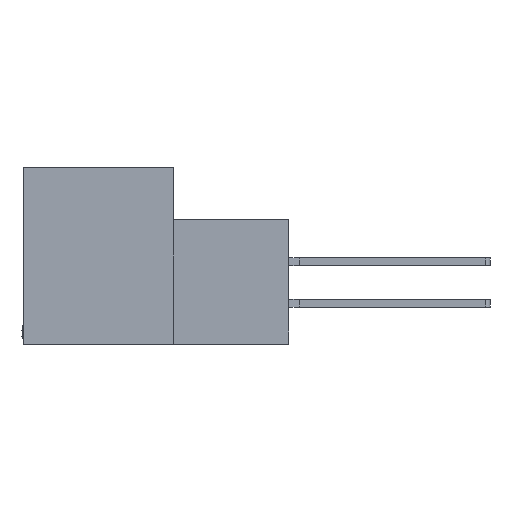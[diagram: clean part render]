
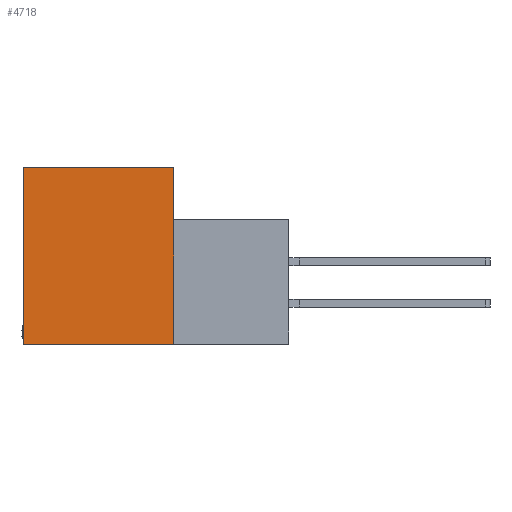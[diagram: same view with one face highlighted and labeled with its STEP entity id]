
A CAD part, left-side view. The second image highlights one B-rep face of the part: STEP entity #4718.
In plain terms, the highlighted planar face has unit normal (-1, 0, 0).
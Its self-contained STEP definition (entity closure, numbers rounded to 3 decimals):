
#235 = DIRECTION ( 'NONE',  ( 0., 0., 1. ) ) ;
#270 = VECTOR ( 'NONE', #8214, 1000. ) ;
#2529 = VERTEX_POINT ( 'NONE', #7531 ) ;
#2599 = AXIS2_PLACEMENT_3D ( 'NONE', #23667, #19995, #5098 ) ;
#4718 = ADVANCED_FACE ( 'NONE', ( #18733 ), #21499, .F. ) ;
#5098 = DIRECTION ( 'NONE',  ( 0., 0., -1. ) ) ;
#5476 = EDGE_CURVE ( 'NONE', #12645, #7682, #20450, .T. ) ;
#7056 = DIRECTION ( 'NONE',  ( 0., 1., 0. ) ) ;
#7314 = CARTESIAN_POINT ( 'NONE',  ( 0., 11.506, 0. ) ) ;
#7531 = CARTESIAN_POINT ( 'NONE',  ( 0., 11.506, -13.487 ) ) ;
#7675 = CARTESIAN_POINT ( 'NONE',  ( 0., 0., 0. ) ) ;
#7682 = VERTEX_POINT ( 'NONE', #7675 ) ;
#7828 = LINE ( 'NONE', #21684, #22513 ) ;
#8214 = DIRECTION ( 'NONE',  ( 0., -1., 0. ) ) ;
#8284 = CARTESIAN_POINT ( 'NONE',  ( 0., 11.506, 0. ) ) ;
#9219 = EDGE_LOOP ( 'NONE', ( #10697, #18334, #13505, #21819 ) ) ;
#9712 = CARTESIAN_POINT ( 'NONE',  ( 0., 0., 0. ) ) ;
#10315 = EDGE_CURVE ( 'NONE', #12982, #2529, #7828, .T. ) ;
#10697 = ORIENTED_EDGE ( 'NONE', *, *, #10315, .F. ) ;
#11489 = EDGE_CURVE ( 'NONE', #7682, #12982, #21360, .T. ) ;
#11737 = DIRECTION ( 'NONE',  ( 0., 0., -1. ) ) ;
#11888 = CARTESIAN_POINT ( 'NONE',  ( 0., 0., -13.487 ) ) ;
#12155 = VECTOR ( 'NONE', #11737, 1000. ) ;
#12645 = VERTEX_POINT ( 'NONE', #7314 ) ;
#12982 = VERTEX_POINT ( 'NONE', #11888 ) ;
#13505 = ORIENTED_EDGE ( 'NONE', *, *, #5476, .F. ) ;
#17398 = VECTOR ( 'NONE', #235, 1000. ) ;
#17971 = LINE ( 'NONE', #20854, #17398 ) ;
#18334 = ORIENTED_EDGE ( 'NONE', *, *, #11489, .F. ) ;
#18733 = FACE_OUTER_BOUND ( 'NONE', #9219, .T. ) ;
#19995 = DIRECTION ( 'NONE',  ( 1., 0., 0. ) ) ;
#20450 = LINE ( 'NONE', #8284, #270 ) ;
#20854 = CARTESIAN_POINT ( 'NONE',  ( 0., 11.506, -13.487 ) ) ;
#21169 = EDGE_CURVE ( 'NONE', #2529, #12645, #17971, .T. ) ;
#21360 = LINE ( 'NONE', #9712, #12155 ) ;
#21499 = PLANE ( 'NONE',  #2599 ) ;
#21684 = CARTESIAN_POINT ( 'NONE',  ( 0., -8.814, -13.487 ) ) ;
#21819 = ORIENTED_EDGE ( 'NONE', *, *, #21169, .F. ) ;
#22513 = VECTOR ( 'NONE', #7056, 1000. ) ;
#23667 = CARTESIAN_POINT ( 'NONE',  ( 0., 0., 0. ) ) ;
